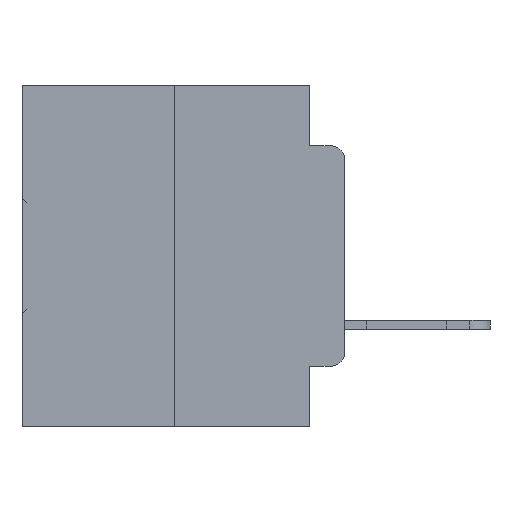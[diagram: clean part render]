
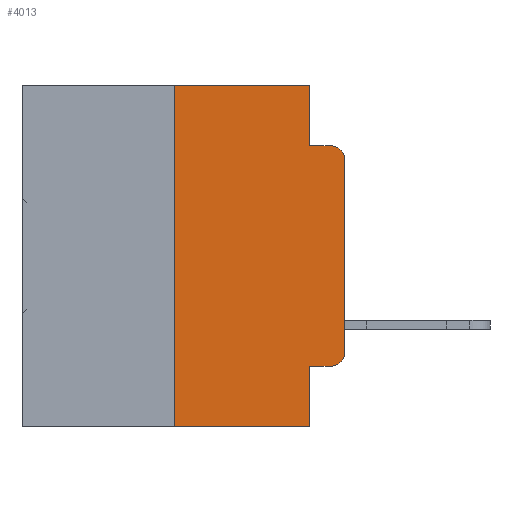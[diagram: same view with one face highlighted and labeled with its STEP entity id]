
A CAD part, left-side view. The second image highlights one B-rep face of the part: STEP entity #4013.
In plain terms, the highlighted planar face has unit normal (-1, 0, 0).
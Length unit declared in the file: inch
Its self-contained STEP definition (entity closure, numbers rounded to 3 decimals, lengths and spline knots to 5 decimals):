
#89 = CARTESIAN_POINT ( 'NONE',  ( 0., 0.25, 0. ) ) ;
#95 = AXIS2_PLACEMENT_3D ( 'NONE', #4992, #15354, #15464 ) ;
#185 = ORIENTED_EDGE ( 'NONE', *, *, #20553, .F. ) ;
#533 = DIRECTION ( 'NONE',  ( 0., 0., 1. ) ) ;
#837 = LINE ( 'NONE', #25921, #13262 ) ;
#935 = EDGE_CURVE ( 'NONE', #14074, #17512, #18340, .T. ) ;
#1259 = CARTESIAN_POINT ( 'NONE',  ( 0., 0.473, -0.5 ) ) ;
#1577 = ORIENTED_EDGE ( 'NONE', *, *, #17318, .T. ) ;
#1990 = LINE ( 'NONE', #13739, #15093 ) ;
#2448 = VECTOR ( 'NONE', #23184, 39.37008 ) ;
#2497 = ORIENTED_EDGE ( 'NONE', *, *, #935, .F. ) ;
#2697 = AXIS2_PLACEMENT_3D ( 'NONE', #15627, #32076, #18062 ) ;
#2996 = VERTEX_POINT ( 'NONE', #28265 ) ;
#3722 = DIRECTION ( 'NONE',  ( 0., -1., 0. ) ) ;
#4013 = ADVANCED_FACE ( 'NONE', ( #23123 ), #4920, .F. ) ;
#4254 = ORIENTED_EDGE ( 'NONE', *, *, #21270, .T. ) ;
#4270 = VECTOR ( 'NONE', #19558, 39.37008 ) ;
#4312 = CARTESIAN_POINT ( 'NONE',  ( 0., 0.051, -0.0885 ) ) ;
#4674 = VECTOR ( 'NONE', #3722, 39.37008 ) ;
#4829 = CARTESIAN_POINT ( 'NONE',  ( 0., 0.25, -0.5 ) ) ;
#4920 = PLANE ( 'NONE',  #95 ) ;
#4927 = CIRCLE ( 'NONE', #2697, 0.02 ) ;
#4992 = CARTESIAN_POINT ( 'NONE',  ( 0., 0.473, 0. ) ) ;
#5451 = VERTEX_POINT ( 'NONE', #19542 ) ;
#5603 = CARTESIAN_POINT ( 'NONE',  ( 0., 0.051, -0.0885 ) ) ;
#6183 = DIRECTION ( 'NONE',  ( 0., -1., 0. ) ) ;
#7263 = VERTEX_POINT ( 'NONE', #9447 ) ;
#8184 = ORIENTED_EDGE ( 'NONE', *, *, #8941, .F. ) ;
#8941 = EDGE_CURVE ( 'NONE', #7263, #5451, #17971, .T. ) ;
#9350 = ORIENTED_EDGE ( 'NONE', *, *, #26882, .T. ) ;
#9447 = CARTESIAN_POINT ( 'NONE',  ( 0., 0.25, 0. ) ) ;
#9549 = VERTEX_POINT ( 'NONE', #21845 ) ;
#9951 = VECTOR ( 'NONE', #24019, 39.37008 ) ;
#10537 = DIRECTION ( 'NONE',  ( 0., 0., -1. ) ) ;
#11019 = CARTESIAN_POINT ( 'NONE',  ( 0., 0.051, 0. ) ) ;
#11867 = VERTEX_POINT ( 'NONE', #14076 ) ;
#11893 = LINE ( 'NONE', #89, #17734 ) ;
#12298 = EDGE_CURVE ( 'NONE', #17859, #2996, #4927, .T. ) ;
#12522 = AXIS2_PLACEMENT_3D ( 'NONE', #28389, #14138, #30745 ) ;
#13066 = CARTESIAN_POINT ( 'NONE',  ( 0., 0.051, 0. ) ) ;
#13262 = VECTOR ( 'NONE', #6183, 39.37008 ) ;
#13481 = DIRECTION ( 'NONE',  ( 0., 0., 1. ) ) ;
#13610 = VECTOR ( 'NONE', #10537, 39.37008 ) ;
#13739 = CARTESIAN_POINT ( 'NONE',  ( 0., 0., 0. ) ) ;
#14074 = VERTEX_POINT ( 'NONE', #5603 ) ;
#14076 = CARTESIAN_POINT ( 'NONE',  ( 0., 0., -0.1085 ) ) ;
#14138 = DIRECTION ( 'NONE',  ( -1., 0., 0. ) ) ;
#14416 = LINE ( 'NONE', #13066, #13610 ) ;
#14590 = ORIENTED_EDGE ( 'NONE', *, *, #12298, .T. ) ;
#14679 = CARTESIAN_POINT ( 'NONE',  ( 0., 0.02, -0.0885 ) ) ;
#15093 = VECTOR ( 'NONE', #533, 39.37008 ) ;
#15354 = DIRECTION ( 'NONE',  ( 1., 0., 0. ) ) ;
#15464 = DIRECTION ( 'NONE',  ( 0., 0., -1. ) ) ;
#15627 = CARTESIAN_POINT ( 'NONE',  ( 0., 0.02, -0.3915 ) ) ;
#15898 = EDGE_LOOP ( 'NONE', ( #4254, #16134, #2497, #21699, #8184, #31031, #9350, #185, #1577, #14590 ) ) ;
#16134 = ORIENTED_EDGE ( 'NONE', *, *, #29848, .T. ) ;
#17318 = EDGE_CURVE ( 'NONE', #26463, #17859, #837, .T. ) ;
#17512 = VERTEX_POINT ( 'NONE', #14679 ) ;
#17734 = VECTOR ( 'NONE', #13481, 39.37008 ) ;
#17859 = VERTEX_POINT ( 'NONE', #27710 ) ;
#17971 = LINE ( 'NONE', #21974, #4270 ) ;
#18062 = DIRECTION ( 'NONE',  ( 0., 0., -1. ) ) ;
#18340 = LINE ( 'NONE', #4312, #4674 ) ;
#19542 = CARTESIAN_POINT ( 'NONE',  ( 0., 0.051, 0. ) ) ;
#19558 = DIRECTION ( 'NONE',  ( 0., -1., 0. ) ) ;
#20553 = EDGE_CURVE ( 'NONE', #26463, #9549, #23381, .T. ) ;
#20952 = VERTEX_POINT ( 'NONE', #4829 ) ;
#21270 = EDGE_CURVE ( 'NONE', #2996, #11867, #1990, .T. ) ;
#21699 = ORIENTED_EDGE ( 'NONE', *, *, #31471, .F. ) ;
#21845 = CARTESIAN_POINT ( 'NONE',  ( 0., 0.051, -0.5 ) ) ;
#21974 = CARTESIAN_POINT ( 'NONE',  ( 0., 0.473, 0. ) ) ;
#22078 = EDGE_CURVE ( 'NONE', #20952, #7263, #11893, .T. ) ;
#23123 = FACE_OUTER_BOUND ( 'NONE', #15898, .T. ) ;
#23184 = DIRECTION ( 'NONE',  ( 0., 0., -1. ) ) ;
#23381 = LINE ( 'NONE', #11019, #2448 ) ;
#23697 = LINE ( 'NONE', #1259, #9951 ) ;
#24019 = DIRECTION ( 'NONE',  ( 0., -1., 0. ) ) ;
#25921 = CARTESIAN_POINT ( 'NONE',  ( 0., 0.051, -0.4115 ) ) ;
#26463 = VERTEX_POINT ( 'NONE', #31983 ) ;
#26882 = EDGE_CURVE ( 'NONE', #20952, #9549, #23697, .T. ) ;
#27710 = CARTESIAN_POINT ( 'NONE',  ( 0., 0.02, -0.4115 ) ) ;
#28265 = CARTESIAN_POINT ( 'NONE',  ( 0., 0., -0.3915 ) ) ;
#28389 = CARTESIAN_POINT ( 'NONE',  ( 0., 0.02, -0.1085 ) ) ;
#29848 = EDGE_CURVE ( 'NONE', #11867, #17512, #30211, .T. ) ;
#30211 = CIRCLE ( 'NONE', #12522, 0.02 ) ;
#30745 = DIRECTION ( 'NONE',  ( 0., 0., -1. ) ) ;
#31031 = ORIENTED_EDGE ( 'NONE', *, *, #22078, .F. ) ;
#31471 = EDGE_CURVE ( 'NONE', #5451, #14074, #14416, .T. ) ;
#31983 = CARTESIAN_POINT ( 'NONE',  ( 0., 0.051, -0.4115 ) ) ;
#32076 = DIRECTION ( 'NONE',  ( -1., 0., 0. ) ) ;
